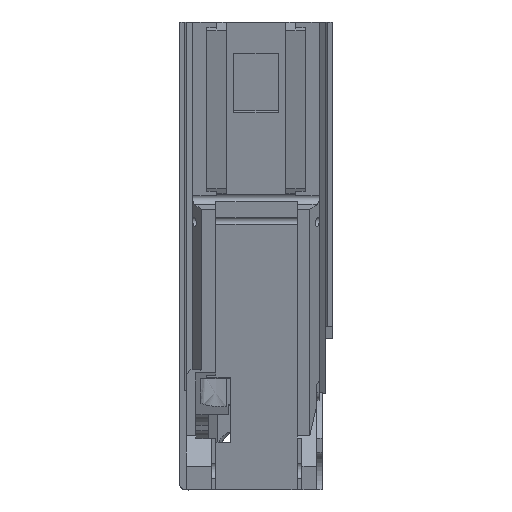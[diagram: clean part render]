
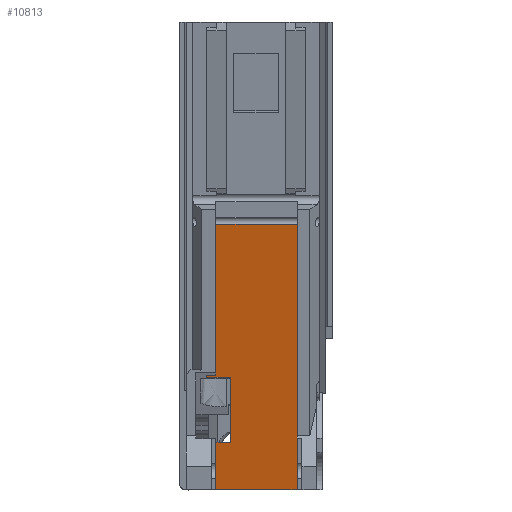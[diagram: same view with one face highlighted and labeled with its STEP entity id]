
A CAD part, front view. The second image highlights one B-rep face of the part: STEP entity #10813.
In plain terms, the highlighted planar face has unit normal (0, -0.966, -0.261).
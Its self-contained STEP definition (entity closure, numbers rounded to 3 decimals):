
#1070=PLANE('',#11471);
#1613=FACE_OUTER_BOUND('',#2207,.T.);
#2207=EDGE_LOOP('',(#9376,#9377,#9378,#9379,#9380,#9381,#9382,#9383,#9384,
#9385,#9386,#9387));
#2657=LINE('',#18426,#3555);
#2955=LINE('',#26921,#3853);
#2970=LINE('',#27022,#3868);
#3063=LINE('',#27362,#3961);
#3069=LINE('',#27376,#3967);
#3091=LINE('',#27418,#3989);
#3092=LINE('',#27420,#3990);
#3093=LINE('',#27421,#3991);
#3094=LINE('',#27423,#3992);
#3095=LINE('',#27425,#3993);
#3096=LINE('',#27426,#3994);
#3097=LINE('',#27427,#3995);
#3555=VECTOR('',#12189,20.6);
#3853=VECTOR('',#12967,4.88);
#3868=VECTOR('',#12994,10.183);
#3961=VECTOR('',#13209,16.7);
#3967=VECTOR('',#13223,1.9);
#3989=VECTOR('',#13273,30.105);
#3990=VECTOR('',#13274,13.811);
#3991=VECTOR('',#13275,4.88);
#3992=VECTOR('',#13276,48.);
#3993=VECTOR('',#13277,2.);
#3994=VECTOR('',#13278,8.476);
#3995=VECTOR('',#13279,2.376);
#4611=VERTEX_POINT('',#18423);
#4612=VERTEX_POINT('',#18425);
#5090=VERTEX_POINT('',#26918);
#5091=VERTEX_POINT('',#26920);
#5109=VERTEX_POINT('',#27021);
#5191=VERTEX_POINT('',#27359);
#5192=VERTEX_POINT('',#27361);
#5195=VERTEX_POINT('',#27374);
#5196=VERTEX_POINT('',#27375);
#5203=VERTEX_POINT('',#27419);
#5204=VERTEX_POINT('',#27422);
#5205=VERTEX_POINT('',#27424);
#5804=EDGE_CURVE('',#4612,#4611,#2657,.T.);
#6532=EDGE_CURVE('',#5091,#5090,#2955,.T.);
#6557=EDGE_CURVE('',#5109,#4612,#2970,.T.);
#6688=EDGE_CURVE('',#5192,#5191,#3063,.T.);
#6695=EDGE_CURVE('',#5195,#5196,#3069,.T.);
#6718=EDGE_CURVE('',#5196,#5091,#3091,.T.);
#6719=EDGE_CURVE('',#5090,#5203,#3092,.T.);
#6720=EDGE_CURVE('',#5109,#5203,#3093,.T.);
#6721=EDGE_CURVE('',#5204,#4611,#3094,.T.);
#6722=EDGE_CURVE('',#5204,#5205,#3095,.T.);
#6723=EDGE_CURVE('',#5192,#5205,#3096,.T.);
#6724=EDGE_CURVE('',#5191,#5195,#3097,.T.);
#9376=ORIENTED_EDGE('',*,*,#6718,.T.);
#9377=ORIENTED_EDGE('',*,*,#6532,.T.);
#9378=ORIENTED_EDGE('',*,*,#6719,.T.);
#9379=ORIENTED_EDGE('',*,*,#6720,.F.);
#9380=ORIENTED_EDGE('',*,*,#6557,.T.);
#9381=ORIENTED_EDGE('',*,*,#5804,.T.);
#9382=ORIENTED_EDGE('',*,*,#6721,.F.);
#9383=ORIENTED_EDGE('',*,*,#6722,.T.);
#9384=ORIENTED_EDGE('',*,*,#6723,.F.);
#9385=ORIENTED_EDGE('',*,*,#6688,.T.);
#9386=ORIENTED_EDGE('',*,*,#6724,.T.);
#9387=ORIENTED_EDGE('',*,*,#6695,.T.);
#10813=ADVANCED_FACE('',(#1613),#1070,.F.);
#11471=AXIS2_PLACEMENT_3D('',#27417,#13271,#13272);
#12189=DIRECTION('',(1.,0.,0.));
#12967=DIRECTION('',(1.,0.,0.));
#12994=DIRECTION('',(0.,0.261,-0.965));
#13209=DIRECTION('',(-1.,0.,0.));
#13223=DIRECTION('',(-1.,0.,0.));
#13271=DIRECTION('center_axis',(0.,0.965,0.261));
#13272=DIRECTION('ref_axis',(0.,-0.261,0.965));
#13273=DIRECTION('',(0.,0.261,-0.965));
#13274=DIRECTION('',(0.,0.261,-0.965));
#13275=DIRECTION('',(1.,0.,0.));
#13276=DIRECTION('',(0.,0.261,-0.965));
#13277=DIRECTION('',(-1.,0.,0.));
#13278=DIRECTION('',(0.,0.261,-0.965));
#13279=DIRECTION('',(0.,0.261,-0.965));
#18423=CARTESIAN_POINT('',(26.125,8.5,0.));
#18425=CARTESIAN_POINT('',(5.525,8.5,0.));
#18426=CARTESIAN_POINT('',(5.525,8.5,0.));
#26918=CARTESIAN_POINT('',(10.405,2.249,23.166));
#26920=CARTESIAN_POINT('',(5.525,2.249,23.166));
#26921=CARTESIAN_POINT('',(5.525,2.249,23.166));
#27021=CARTESIAN_POINT('',(5.525,5.847,9.832));
#27022=CARTESIAN_POINT('',(5.525,5.847,9.832));
#27359=CARTESIAN_POINT('',(7.425,-6.212,54.526));
#27361=CARTESIAN_POINT('',(24.125,-6.212,54.526));
#27362=CARTESIAN_POINT('',(24.125,-6.212,54.526));
#27374=CARTESIAN_POINT('',(7.425,-5.593,52.232));
#27375=CARTESIAN_POINT('',(5.525,-5.593,52.232));
#27376=CARTESIAN_POINT('',(7.425,-5.593,52.232));
#27417=CARTESIAN_POINT('Origin',(0.,-20.677,108.133));
#27418=CARTESIAN_POINT('',(5.525,-5.593,52.232));
#27419=CARTESIAN_POINT('',(10.405,5.847,9.832));
#27420=CARTESIAN_POINT('',(10.405,2.249,23.166));
#27421=CARTESIAN_POINT('',(5.525,5.847,9.832));
#27422=CARTESIAN_POINT('',(26.125,-4.004,46.343));
#27423=CARTESIAN_POINT('',(26.125,-4.004,46.343));
#27424=CARTESIAN_POINT('',(24.125,-4.004,46.343));
#27425=CARTESIAN_POINT('',(26.125,-4.004,46.343));
#27426=CARTESIAN_POINT('',(24.125,-6.212,54.526));
#27427=CARTESIAN_POINT('',(7.425,-6.212,54.526));
